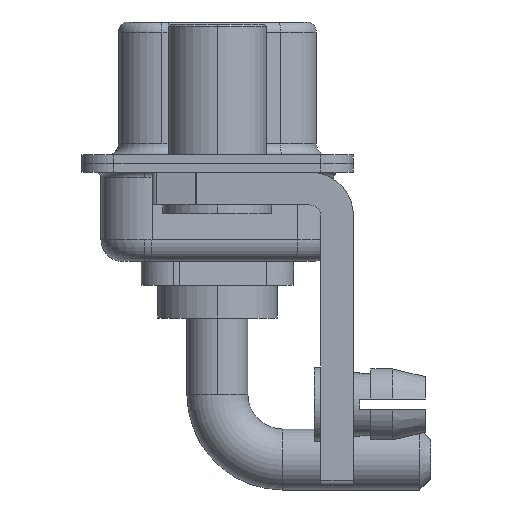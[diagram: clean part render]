
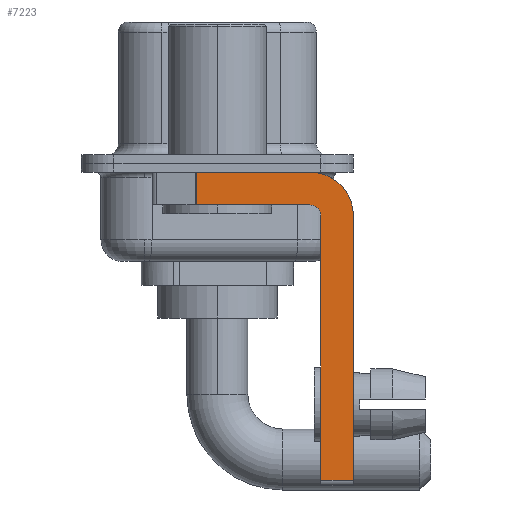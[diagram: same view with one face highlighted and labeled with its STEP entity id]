
A CAD part, left-side view. The second image highlights one B-rep face of the part: STEP entity #7223.
In plain terms, the highlighted planar face has unit normal (-1, 0, 0).
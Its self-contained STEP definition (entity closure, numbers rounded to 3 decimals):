
#264 = EDGE_CURVE ( 'NONE', #15291, #3867, #3021, .T. ) ;
#385 = DIRECTION ( 'NONE',  ( 0., 0., -1. ) ) ;
#594 = CARTESIAN_POINT ( 'NONE',  ( -2.9, -4.75, -14.55 ) ) ;
#747 = EDGE_CURVE ( 'NONE', #13310, #15291, #3494, .T. ) ;
#1261 = DIRECTION ( 'NONE',  ( 0., 0., 1. ) ) ;
#1407 = AXIS2_PLACEMENT_3D ( 'NONE', #10179, #14449, #2789 ) ;
#1695 = VECTOR ( 'NONE', #1261, 1000. ) ;
#2442 = ORIENTED_EDGE ( 'NONE', *, *, #13203, .F. ) ;
#2459 = CARTESIAN_POINT ( 'NONE',  ( -2.9, -4.25, -14.55 ) ) ;
#2789 = DIRECTION ( 'NONE',  ( 0., 0., 1. ) ) ;
#2824 = EDGE_CURVE ( 'NONE', #11999, #6570, #8728, .T. ) ;
#2878 = ORIENTED_EDGE ( 'NONE', *, *, #264, .F. ) ;
#3021 = LINE ( 'NONE', #8846, #17813 ) ;
#3456 = VECTOR ( 'NONE', #5462, 1000. ) ;
#3494 = CIRCLE ( 'NONE', #6573, 2. ) ;
#3603 = EDGE_CURVE ( 'NONE', #15558, #17057, #19132, .T. ) ;
#3639 = ORIENTED_EDGE ( 'NONE', *, *, #2824, .T. ) ;
#3867 = VERTEX_POINT ( 'NONE', #6071 ) ;
#3983 = CARTESIAN_POINT ( 'NONE',  ( -2.9, -4.75, -14.8 ) ) ;
#4201 = LINE ( 'NONE', #2459, #3456 ) ;
#4474 = VECTOR ( 'NONE', #14853, 1000. ) ;
#4747 = DIRECTION ( 'NONE',  ( 1., 0., 0. ) ) ;
#5462 = DIRECTION ( 'NONE',  ( 0., -1., 0. ) ) ;
#5522 = DIRECTION ( 'NONE',  ( 1., 0., 0. ) ) ;
#5800 = CARTESIAN_POINT ( 'NONE',  ( -2.9, 0.978, -1.9 ) ) ;
#6011 = FACE_OUTER_BOUND ( 'NONE', #15317, .T. ) ;
#6071 = CARTESIAN_POINT ( 'NONE',  ( -2.9, -6.25, -14.55 ) ) ;
#6193 = CARTESIAN_POINT ( 'NONE',  ( -2.9, -4.25, -0.4 ) ) ;
#6570 = VERTEX_POINT ( 'NONE', #14702 ) ;
#6573 = AXIS2_PLACEMENT_3D ( 'NONE', #10201, #5522, #14469 ) ;
#7223 = ADVANCED_FACE ( 'NONE', ( #6011 ), #11971, .F. ) ;
#7454 = ORIENTED_EDGE ( 'NONE', *, *, #10776, .F. ) ;
#7550 = ORIENTED_EDGE ( 'NONE', *, *, #15971, .T. ) ;
#8335 = ORIENTED_EDGE ( 'NONE', *, *, #11790, .F. ) ;
#8728 = LINE ( 'NONE', #5800, #4474 ) ;
#8846 = CARTESIAN_POINT ( 'NONE',  ( -2.9, -6.25, -2.4 ) ) ;
#9311 = CARTESIAN_POINT ( 'NONE',  ( -2.9, -4.25, -2.4 ) ) ;
#9358 = ORIENTED_EDGE ( 'NONE', *, *, #3603, .F. ) ;
#9686 = CARTESIAN_POINT ( 'NONE',  ( -2.9, -4.75, -2.4 ) ) ;
#9914 = LINE ( 'NONE', #3983, #1695 ) ;
#10179 = CARTESIAN_POINT ( 'NONE',  ( -2.9, -4.25, -2.4 ) ) ;
#10201 = CARTESIAN_POINT ( 'NONE',  ( -2.9, -4.25, -2.4 ) ) ;
#10213 = VECTOR ( 'NONE', #14380, 1000. ) ;
#10321 = VERTEX_POINT ( 'NONE', #594 ) ;
#10776 = EDGE_CURVE ( 'NONE', #11999, #13310, #18622, .T. ) ;
#11106 = AXIS2_PLACEMENT_3D ( 'NONE', #9311, #4747, #385 ) ;
#11790 = EDGE_CURVE ( 'NONE', #10321, #15558, #9914, .T. ) ;
#11971 = PLANE ( 'NONE',  #11106 ) ;
#11999 = VERTEX_POINT ( 'NONE', #16228 ) ;
#12596 = DIRECTION ( 'NONE',  ( 0., -1., 0. ) ) ;
#12782 = CARTESIAN_POINT ( 'NONE',  ( -2.9, 3., -0.4 ) ) ;
#12831 = LINE ( 'NONE', #14572, #10213 ) ;
#12954 = ORIENTED_EDGE ( 'NONE', *, *, #747, .F. ) ;
#13203 = EDGE_CURVE ( 'NONE', #17057, #6570, #12831, .T. ) ;
#13310 = VERTEX_POINT ( 'NONE', #6193 ) ;
#14380 = DIRECTION ( 'NONE',  ( 0., 1., 0. ) ) ;
#14449 = DIRECTION ( 'NONE',  ( -1., 0., 0. ) ) ;
#14469 = DIRECTION ( 'NONE',  ( 0., 0., -1. ) ) ;
#14572 = CARTESIAN_POINT ( 'NONE',  ( -2.9, -4.25, -1.9 ) ) ;
#14702 = CARTESIAN_POINT ( 'NONE',  ( -2.9, 0.978, -1.9 ) ) ;
#14853 = DIRECTION ( 'NONE',  ( 0., 0., -1. ) ) ;
#15291 = VERTEX_POINT ( 'NONE', #16478 ) ;
#15317 = EDGE_LOOP ( 'NONE', ( #7454, #3639, #2442, #9358, #8335, #7550, #2878, #12954 ) ) ;
#15558 = VERTEX_POINT ( 'NONE', #9686 ) ;
#15971 = EDGE_CURVE ( 'NONE', #10321, #3867, #4201, .T. ) ;
#16228 = CARTESIAN_POINT ( 'NONE',  ( -2.9, 0.978, -0.4 ) ) ;
#16478 = CARTESIAN_POINT ( 'NONE',  ( -2.9, -6.25, -2.4 ) ) ;
#17057 = VERTEX_POINT ( 'NONE', #17147 ) ;
#17136 = VECTOR ( 'NONE', #12596, 1000. ) ;
#17147 = CARTESIAN_POINT ( 'NONE',  ( -2.9, -4.25, -1.9 ) ) ;
#17703 = DIRECTION ( 'NONE',  ( 0., 0., -1. ) ) ;
#17813 = VECTOR ( 'NONE', #17703, 1000. ) ;
#18622 = LINE ( 'NONE', #12782, #17136 ) ;
#19132 = CIRCLE ( 'NONE', #1407, 0.5 ) ;
